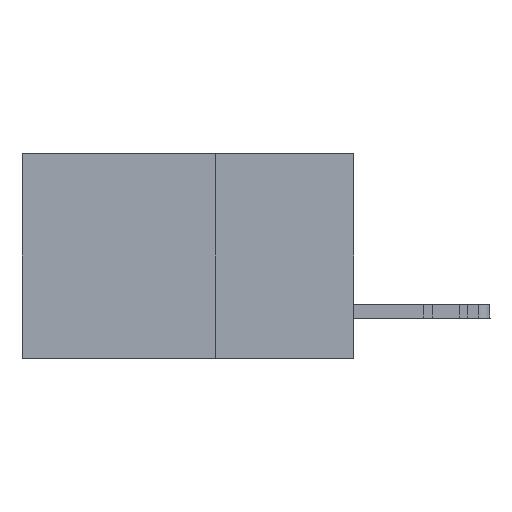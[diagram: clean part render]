
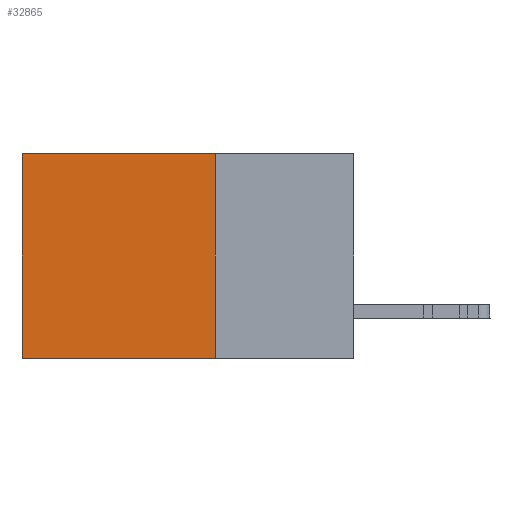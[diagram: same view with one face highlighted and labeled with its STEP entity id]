
A CAD part, left-side view. The second image highlights one B-rep face of the part: STEP entity #32865.
In plain terms, the highlighted planar face has unit normal (-1, 0, 0).
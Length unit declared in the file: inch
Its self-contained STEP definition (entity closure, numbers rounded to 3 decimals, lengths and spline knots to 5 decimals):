
#963 = ORIENTED_EDGE ( 'NONE', *, *, #21323, .T. ) ;
#1240 = CARTESIAN_POINT ( 'NONE',  ( 0.2875, 0.25, -0.37 ) ) ;
#4147 = CARTESIAN_POINT ( 'NONE',  ( 0.2875, 0.6, 0. ) ) ;
#7140 = EDGE_CURVE ( 'NONE', #46028, #27526, #8324, .T. ) ;
#8236 = DIRECTION ( 'NONE',  ( 0., 1., 0. ) ) ;
#8324 = LINE ( 'NONE', #14936, #37335 ) ;
#9109 = PLANE ( 'NONE',  #36982 ) ;
#10741 = DIRECTION ( 'NONE',  ( 0., 0., -1. ) ) ;
#10822 = ORIENTED_EDGE ( 'NONE', *, *, #17368, .T. ) ;
#12145 = LINE ( 'NONE', #40161, #38790 ) ;
#14086 = DIRECTION ( 'NONE',  ( 0., 1., 0. ) ) ;
#14710 = CARTESIAN_POINT ( 'NONE',  ( 0.2875, 0.25, 0. ) ) ;
#14936 = CARTESIAN_POINT ( 'NONE',  ( 0.2875, 0.25, 0. ) ) ;
#16515 = DIRECTION ( 'NONE',  ( 1., 0., 0. ) ) ;
#16695 = CARTESIAN_POINT ( 'NONE',  ( 0.2875, 0.25, 0. ) ) ;
#17368 = EDGE_CURVE ( 'NONE', #44711, #24094, #12145, .T. ) ;
#18800 = DIRECTION ( 'NONE',  ( 0., 0., -1. ) ) ;
#19841 = EDGE_LOOP ( 'NONE', ( #10822, #46150, #22778, #963 ) ) ;
#20414 = DIRECTION ( 'NONE',  ( 0., 0., -1. ) ) ;
#21323 = EDGE_CURVE ( 'NONE', #46028, #44711, #37016, .T. ) ;
#22374 = CARTESIAN_POINT ( 'NONE',  ( 0.2875, 0.6, -0.37 ) ) ;
#22379 = CARTESIAN_POINT ( 'NONE',  ( 0.2875, 0.25, 0. ) ) ;
#22778 = ORIENTED_EDGE ( 'NONE', *, *, #7140, .F. ) ;
#24094 = VERTEX_POINT ( 'NONE', #22374 ) ;
#26445 = EDGE_CURVE ( 'NONE', #27526, #24094, #34167, .T. ) ;
#27526 = VERTEX_POINT ( 'NONE', #43659 ) ;
#32865 = ADVANCED_FACE ( 'NONE', ( #42207 ), #9109, .F. ) ;
#34167 = LINE ( 'NONE', #1240, #47992 ) ;
#36982 = AXIS2_PLACEMENT_3D ( 'NONE', #16695, #16515, #20414 ) ;
#37016 = LINE ( 'NONE', #22379, #38295 ) ;
#37335 = VECTOR ( 'NONE', #18800, 39.37008 ) ;
#38295 = VECTOR ( 'NONE', #14086, 39.37008 ) ;
#38790 = VECTOR ( 'NONE', #10741, 39.37008 ) ;
#40161 = CARTESIAN_POINT ( 'NONE',  ( 0.2875, 0.6, 0. ) ) ;
#42207 = FACE_OUTER_BOUND ( 'NONE', #19841, .T. ) ;
#43659 = CARTESIAN_POINT ( 'NONE',  ( 0.2875, 0.25, -0.37 ) ) ;
#44711 = VERTEX_POINT ( 'NONE', #4147 ) ;
#46028 = VERTEX_POINT ( 'NONE', #14710 ) ;
#46150 = ORIENTED_EDGE ( 'NONE', *, *, #26445, .F. ) ;
#47992 = VECTOR ( 'NONE', #8236, 39.37008 ) ;
